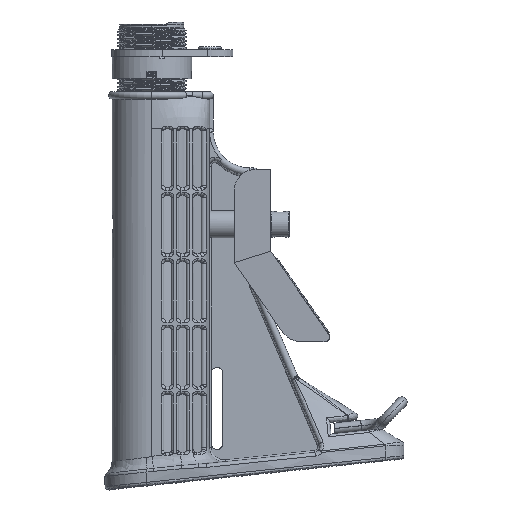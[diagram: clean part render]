
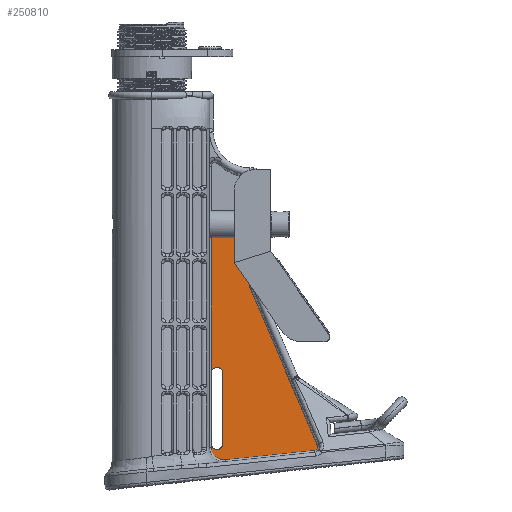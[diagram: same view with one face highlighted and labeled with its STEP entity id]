
A CAD part, left-side view. The second image highlights one B-rep face of the part: STEP entity #250810.
In plain terms, the highlighted planar face has unit normal (-1, 0, 0).
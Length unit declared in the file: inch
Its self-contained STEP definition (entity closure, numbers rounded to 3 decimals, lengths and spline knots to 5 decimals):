
#3777 = ORIENTED_EDGE ( 'NONE', *, *, #173145, .F. ) ;
#4662 = VERTEX_POINT ( 'NONE', #170584 ) ;
#5215 = CARTESIAN_POINT ( 'NONE',  ( -0.0575, -1.23076, -6.06058 ) ) ;
#7054 = ORIENTED_EDGE ( 'NONE', *, *, #154112, .F. ) ;
#8356 = CARTESIAN_POINT ( 'NONE',  ( -0.0575, -1.66875, -2.49043 ) ) ;
#8663 = DIRECTION ( 'NONE',  ( 0., 0., -1. ) ) ;
#10635 = CARTESIAN_POINT ( 'NONE',  ( -0.0575, -1.21201, 0. ) ) ;
#10793 = CARTESIAN_POINT ( 'NONE',  ( -0.0575, -1.66875, -3.3064 ) ) ;
#11241 = EDGE_CURVE ( 'NONE', #185048, #50499, #237045, .T. ) ;
#18140 = CARTESIAN_POINT ( 'NONE',  ( -0.0575, 0., 0. ) ) ;
#19849 = VERTEX_POINT ( 'NONE', #84833 ) ;
#22021 = ORIENTED_EDGE ( 'NONE', *, *, #167723, .F. ) ;
#25299 = DIRECTION ( 'NONE',  ( 0., 0., -1. ) ) ;
#31650 = VECTOR ( 'NONE', #163228, 39.37008 ) ;
#32372 = EDGE_CURVE ( 'NONE', #74230, #195380, #133529, .T. ) ;
#33400 = ORIENTED_EDGE ( 'NONE', *, *, #150825, .F. ) ;
#33623 = CARTESIAN_POINT ( 'NONE',  ( -0.0575, -1.02463, -6.05036 ) ) ;
#38303 = DIRECTION ( 'NONE',  ( 0., 0., -1. ) ) ;
#38765 = CARTESIAN_POINT ( 'NONE',  ( -0.0575, -1.79375, -3.3064 ) ) ;
#39269 = CARTESIAN_POINT ( 'NONE',  ( -0.0575, -1.67881, -3.35552 ) ) ;
#39642 = AXIS2_PLACEMENT_3D ( 'NONE', #213172, #92582, #233170 ) ;
#41146 = CARTESIAN_POINT ( 'NONE',  ( -0.0575, -1.67881, -3.35552 ) ) ;
#42029 = DIRECTION ( 'NONE',  ( 0., -0.393, -0.92 ) ) ;
#42376 = DIRECTION ( 'NONE',  ( 0., -1., 0. ) ) ;
#42551 = CARTESIAN_POINT ( 'NONE',  ( -0.0575, -1.01201, 0. ) ) ;
#45917 = ORIENTED_EDGE ( 'NONE', *, *, #86697, .F. ) ;
#50052 = EDGE_LOOP ( 'NONE', ( #3777, #107467, #121498, #7054, #247576, #58811, #33400, #22021, #45917, #112672, #121812, #243693, #191813 ) ) ;
#50499 = VERTEX_POINT ( 'NONE', #218731 ) ;
#53821 = CARTESIAN_POINT ( 'NONE',  ( -0.0575, -1.05055, -6.07997 ) ) ;
#53940 = CARTESIAN_POINT ( 'NONE',  ( -0.0575, -2.7717, -6.11857 ) ) ;
#54309 = EDGE_CURVE ( 'NONE', #242175, #19849, #245021, .T. ) ;
#58811 = ORIENTED_EDGE ( 'NONE', *, *, #208170, .F. ) ;
#58931 = DIRECTION ( 'NONE',  ( 0., -1., 0. ) ) ;
#61884 = VECTOR ( 'NONE', #42376, 39.37008 ) ;
#68221 = LINE ( 'NONE', #102266, #61884 ) ;
#71482 = VERTEX_POINT ( 'NONE', #222687 ) ;
#74080 = CARTESIAN_POINT ( 'NONE',  ( -0.0575, -1.08583, -6.0974 ) ) ;
#74230 = VERTEX_POINT ( 'NONE', #8356 ) ;
#77197 = VECTOR ( 'NONE', #150511, 39.37008 ) ;
#83611 = LINE ( 'NONE', #10635, #77197 ) ;
#84833 = CARTESIAN_POINT ( 'NONE',  ( -0.0575, -2.82264, -6.03185 ) ) ;
#86404 = CARTESIAN_POINT ( 'NONE',  ( -0.0575, -1.01201, -6. ) ) ;
#86697 = EDGE_CURVE ( 'NONE', #257556, #4662, #129741, .T. ) ;
#86841 = EDGE_CURVE ( 'NONE', #259135, #220103, #151691, .T. ) ;
#92582 = DIRECTION ( 'NONE',  ( -1., 0., 0. ) ) ;
#92659 = CARTESIAN_POINT ( 'NONE',  ( -0.0575, -1.01201, -6. ) ) ;
#94394 = CARTESIAN_POINT ( 'NONE',  ( -0.0575, -1.11201, -6.1 ) ) ;
#95382 = DIRECTION ( 'NONE',  ( 0., 0.995, -0.105 ) ) ;
#97376 = CARTESIAN_POINT ( 'NONE',  ( -0.0575, -1.11201, -6.1 ) ) ;
#99149 = CARTESIAN_POINT ( 'NONE',  ( -0.0575, -1.21201, -4.8 ) ) ;
#99629 = CIRCLE ( 'NONE', #39642, 0.1 ) ;
#102266 = CARTESIAN_POINT ( 'NONE',  ( -0.0575, -1.7625, -2.49043 ) ) ;
#104250 = LINE ( 'NONE', #42551, #31650 ) ;
#107467 = ORIENTED_EDGE ( 'NONE', *, *, #86841, .F. ) ;
#112672 = ORIENTED_EDGE ( 'NONE', *, *, #121915, .F. ) ;
#118460 = PLANE ( 'NONE',  #185664 ) ;
#119857 = CARTESIAN_POINT ( 'NONE',  ( -0.0575, -1.66875, 0. ) ) ;
#120876 = CARTESIAN_POINT ( 'NONE',  ( -0.0575, -1.01201, -1.27025 ) ) ;
#121498 = ORIENTED_EDGE ( 'NONE', *, *, #175077, .F. ) ;
#121604 = DIRECTION ( 'NONE',  ( 0., 0., -1. ) ) ;
#121812 = ORIENTED_EDGE ( 'NONE', *, *, #54309, .F. ) ;
#121915 = EDGE_CURVE ( 'NONE', #19849, #257556, #237563, .T. ) ;
#126432 = VECTOR ( 'NONE', #221107, 39.37008 ) ;
#129135 = DIRECTION ( 'NONE',  ( 1., 0., 0. ) ) ;
#129741 = LINE ( 'NONE', #53940, #176889 ) ;
#133529 = LINE ( 'NONE', #119857, #180713 ) ;
#145883 = DIRECTION ( 'NONE',  ( 1., 0., 0. ) ) ;
#150511 = DIRECTION ( 'NONE',  ( 0., 0., 1. ) ) ;
#150825 = EDGE_CURVE ( 'NONE', #71482, #215738, #104250, .T. ) ;
#150904 = VECTOR ( 'NONE', #42029, 39.37008 ) ;
#151691 = LINE ( 'NONE', #120876, #126432 ) ;
#154112 = EDGE_CURVE ( 'NONE', #50499, #256430, #83611, .T. ) ;
#154311 = CARTESIAN_POINT ( 'NONE',  ( -0.0575, -1.01461, -6.02617 ) ) ;
#158938 = DIRECTION ( 'NONE',  ( 1., 0., 0. ) ) ;
#163228 = DIRECTION ( 'NONE',  ( 0., 0., 1. ) ) ;
#167723 = EDGE_CURVE ( 'NONE', #4662, #71482, #173860, .T. ) ;
#168009 = FACE_OUTER_BOUND ( 'NONE', #50052, .T. ) ;
#170584 = CARTESIAN_POINT ( 'NONE',  ( -0.0575, -1.25362, -6.27813 ) ) ;
#172369 = EDGE_CURVE ( 'NONE', #195380, #242175, #197555, .T. ) ;
#172492 = CARTESIAN_POINT ( 'NONE',  ( -0.0575, -1.21201, -6. ) ) ;
#172551 = CARTESIAN_POINT ( 'NONE',  ( -0.0575, -1.21201, -6.01309 ) ) ;
#172759 = CARTESIAN_POINT ( 'NONE',  ( -0.0575, -1.2094, -6.02617 ) ) ;
#172797 = CARTESIAN_POINT ( 'NONE',  ( -0.0575, -1.19939, -6.05036 ) ) ;
#173117 = CARTESIAN_POINT ( 'NONE',  ( -0.0575, -1.19197, -6.06145 ) ) ;
#173145 = EDGE_CURVE ( 'NONE', #220103, #74230, #68221, .T. ) ;
#173355 = CARTESIAN_POINT ( 'NONE',  ( -0.0575, -1.17346, -6.07997 ) ) ;
#173414 = CARTESIAN_POINT ( 'NONE',  ( -0.0575, -1.16237, -6.08738 ) ) ;
#173638 = CARTESIAN_POINT ( 'NONE',  ( -0.0575, -1.11201, -6.1 ) ) ;
#173860 = CIRCLE ( 'NONE', #173934, 0.21875 ) ;
#173934 = AXIS2_PLACEMENT_3D ( 'NONE', #5215, #145883, #25299 ) ;
#174266 = CARTESIAN_POINT ( 'NONE',  ( -0.0575, -1.1251, -6.1 ) ) ;
#174535 = CARTESIAN_POINT ( 'NONE',  ( -0.0575, -1.03204, -6.06145 ) ) ;
#175077 = EDGE_CURVE ( 'NONE', #256430, #259135, #99629, .T. ) ;
#176889 = VECTOR ( 'NONE', #95382, 39.37008 ) ;
#177109 = CARTESIAN_POINT ( 'NONE',  ( -0.0575, -1.13818, -6.0974 ) ) ;
#179663 = DIRECTION ( 'NONE',  ( -1., 0., 0. ) ) ;
#180713 = VECTOR ( 'NONE', #121604, 39.37008 ) ;
#185048 = VERTEX_POINT ( 'NONE', #97376 ) ;
#185664 = AXIS2_PLACEMENT_3D ( 'NONE', #18140, #158938, #38303 ) ;
#191813 = ORIENTED_EDGE ( 'NONE', *, *, #32372, .F. ) ;
#194724 = CARTESIAN_POINT ( 'NONE',  ( -0.0575, -1.06165, -6.08738 ) ) ;
#195380 = VERTEX_POINT ( 'NONE', #10793 ) ;
#197429 = B_SPLINE_CURVE_WITH_KNOTS ( 'NONE', 3,
 ( #92659, #253304, #154311, #33623, #174535, #53821, #194724, #74080, #214943, #94394 ),
 .UNSPECIFIED., .F., .F.,
 ( 4, 2, 2, 2, 4 ),
 ( 0., 0.25, 0.5, 0.75, 1. ),
 .UNSPECIFIED. ) ;
#197555 = CIRCLE ( 'NONE', #258135, 0.125 ) ;
#204596 = AXIS2_PLACEMENT_3D ( 'NONE', #249294, #129135, #8663 ) ;
#208170 = EDGE_CURVE ( 'NONE', #215738, #185048, #197429, .T. ) ;
#213172 = CARTESIAN_POINT ( 'NONE',  ( -0.0575, -1.11201, -4.8 ) ) ;
#214943 = CARTESIAN_POINT ( 'NONE',  ( -0.0575, -1.09892, -6.1 ) ) ;
#215738 = VERTEX_POINT ( 'NONE', #86404 ) ;
#218731 = CARTESIAN_POINT ( 'NONE',  ( -0.0575, -1.21201, -6. ) ) ;
#220103 = VERTEX_POINT ( 'NONE', #243082 ) ;
#221107 = DIRECTION ( 'NONE',  ( 0., 0., 1. ) ) ;
#222687 = CARTESIAN_POINT ( 'NONE',  ( -0.0575, -1.01201, -6.06058 ) ) ;
#233170 = DIRECTION ( 'NONE',  ( 0., 0., -1. ) ) ;
#237045 = B_SPLINE_CURVE_WITH_KNOTS ( 'NONE', 3,
 ( #173638, #174266, #177109, #173414, #173355, #173117, #172797, #172759, #172551, #172492 ),
 .UNSPECIFIED., .F., .F.,
 ( 4, 2, 2, 2, 4 ),
 ( 0., 0.25, 0.5, 0.75, 1. ),
 .UNSPECIFIED. ) ;
#237563 = CIRCLE ( 'NONE', #204596, 0.0625 ) ;
#240002 = CARTESIAN_POINT ( 'NONE',  ( -0.0575, -1.01201, -4.8 ) ) ;
#242175 = VERTEX_POINT ( 'NONE', #39269 ) ;
#243082 = CARTESIAN_POINT ( 'NONE',  ( -0.0575, -1.01201, -2.49043 ) ) ;
#243693 = ORIENTED_EDGE ( 'NONE', *, *, #172369, .F. ) ;
#245021 = LINE ( 'NONE', #41146, #150904 ) ;
#247576 = ORIENTED_EDGE ( 'NONE', *, *, #11241, .F. ) ;
#247740 = CARTESIAN_POINT ( 'NONE',  ( -0.0575, -2.7717, -6.11857 ) ) ;
#249294 = CARTESIAN_POINT ( 'NONE',  ( -0.0575, -2.76517, -6.05641 ) ) ;
#250810 = ADVANCED_FACE ( 'NONE', ( #168009 ), #118460, .F. ) ;
#253304 = CARTESIAN_POINT ( 'NONE',  ( -0.0575, -1.01201, -6.01309 ) ) ;
#256430 = VERTEX_POINT ( 'NONE', #99149 ) ;
#257556 = VERTEX_POINT ( 'NONE', #247740 ) ;
#258135 = AXIS2_PLACEMENT_3D ( 'NONE', #38765, #179663, #58931 ) ;
#259135 = VERTEX_POINT ( 'NONE', #240002 ) ;
